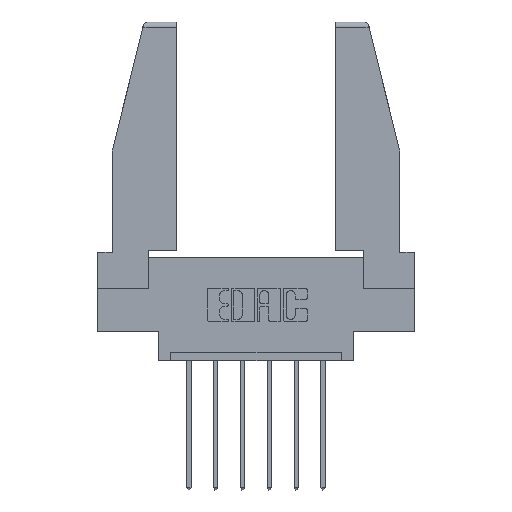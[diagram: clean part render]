
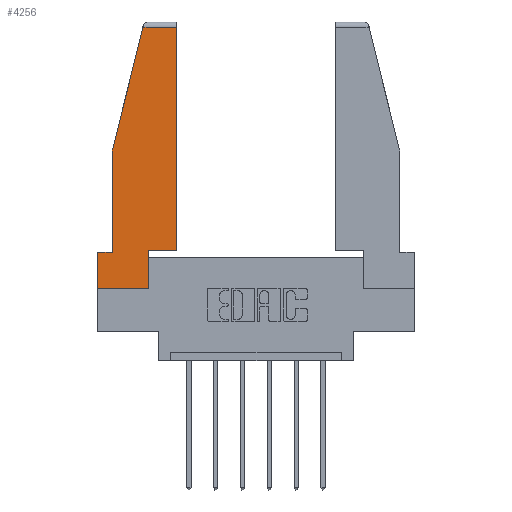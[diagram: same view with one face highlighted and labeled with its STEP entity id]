
A CAD part, top view. The second image highlights one B-rep face of the part: STEP entity #4256.
In plain terms, the highlighted planar face has unit normal (0, 0, 1).
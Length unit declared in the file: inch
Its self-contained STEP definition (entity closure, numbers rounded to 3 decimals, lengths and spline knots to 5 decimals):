
#99 = CARTESIAN_POINT ( 'NONE',  ( 0.297, 0., 0. ) ) ;
#117 = LINE ( 'NONE', #1682, #7533 ) ;
#128 = VERTEX_POINT ( 'NONE', #6214 ) ;
#336 = CARTESIAN_POINT ( 'NONE',  ( 0., 0.21, 0. ) ) ;
#472 = AXIS2_PLACEMENT_3D ( 'NONE', #9961, #860, #3648 ) ;
#632 = CARTESIAN_POINT ( 'NONE',  ( 0.2636, 1.52, 0. ) ) ;
#685 = VECTOR ( 'NONE', #4861, 39.37008 ) ;
#771 = VECTOR ( 'NONE', #7228, 39.37008 ) ;
#847 = CARTESIAN_POINT ( 'NONE',  ( 0.461, 1.52, 0. ) ) ;
#860 = DIRECTION ( 'NONE',  ( 0., 0., 1. ) ) ;
#1025 = VERTEX_POINT ( 'NONE', #632 ) ;
#1047 = EDGE_CURVE ( 'NONE', #10217, #1025, #6096, .T. ) ;
#1245 = DIRECTION ( 'NONE',  ( -1., 0., 0. ) ) ;
#1285 = ORIENTED_EDGE ( 'NONE', *, *, #1887, .T. ) ;
#1404 = ORIENTED_EDGE ( 'NONE', *, *, #4177, .T. ) ;
#1538 = CARTESIAN_POINT ( 'NONE',  ( 0., 1.52, 0. ) ) ;
#1581 = VECTOR ( 'NONE', #1245, 39.37008 ) ;
#1633 = ORIENTED_EDGE ( 'NONE', *, *, #8435, .T. ) ;
#1682 = CARTESIAN_POINT ( 'NONE',  ( 0., 0.21, 0. ) ) ;
#1887 = EDGE_CURVE ( 'NONE', #9279, #9897, #5248, .T. ) ;
#1953 = EDGE_LOOP ( 'NONE', ( #11177, #4930, #1633, #2156, #5743, #11666, #10056, #1285, #1404 ) ) ;
#2156 = ORIENTED_EDGE ( 'NONE', *, *, #6064, .T. ) ;
#2328 = LINE ( 'NONE', #10596, #8303 ) ;
#2685 = DIRECTION ( 'NONE',  ( 0., -1., 0. ) ) ;
#3169 = DIRECTION ( 'NONE',  ( 1., 0., 0. ) ) ;
#3294 = CARTESIAN_POINT ( 'NONE',  ( 0., 0.21, 0. ) ) ;
#3648 = DIRECTION ( 'NONE',  ( 1., 0., 0. ) ) ;
#3787 = DIRECTION ( 'NONE',  ( 0., -1., 0. ) ) ;
#3965 = CARTESIAN_POINT ( 'NONE',  ( 0.297, 0.223, 0. ) ) ;
#3994 = EDGE_CURVE ( 'NONE', #9387, #10217, #2328, .T. ) ;
#4177 = EDGE_CURVE ( 'NONE', #9897, #9387, #7897, .T. ) ;
#4256 = ADVANCED_FACE ( 'NONE', ( #4471 ), #10036, .T. ) ;
#4471 = FACE_OUTER_BOUND ( 'NONE', #1953, .T. ) ;
#4685 = CARTESIAN_POINT ( 'NONE',  ( 0., 0., 0. ) ) ;
#4861 = DIRECTION ( 'NONE',  ( 0., 1., 0. ) ) ;
#4930 = ORIENTED_EDGE ( 'NONE', *, *, #1047, .T. ) ;
#5167 = EDGE_CURVE ( 'NONE', #128, #5883, #8150, .T. ) ;
#5248 = LINE ( 'NONE', #99, #685 ) ;
#5419 = LINE ( 'NONE', #6001, #10674 ) ;
#5514 = CARTESIAN_POINT ( 'NONE',  ( 0.297, 0., 0. ) ) ;
#5559 = DIRECTION ( 'NONE',  ( -1., 0., 0. ) ) ;
#5658 = CARTESIAN_POINT ( 'NONE',  ( 0.461, 0.223, 0. ) ) ;
#5690 = VERTEX_POINT ( 'NONE', #4685 ) ;
#5743 = ORIENTED_EDGE ( 'NONE', *, *, #5167, .T. ) ;
#5883 = VERTEX_POINT ( 'NONE', #3294 ) ;
#6001 = CARTESIAN_POINT ( 'NONE',  ( 0.271, 1.55, 0. ) ) ;
#6064 = EDGE_CURVE ( 'NONE', #8165, #128, #10999, .T. ) ;
#6096 = LINE ( 'NONE', #1538, #6512 ) ;
#6203 = DIRECTION ( 'NONE',  ( 0., 1., 0. ) ) ;
#6214 = CARTESIAN_POINT ( 'NONE',  ( 0.086, 0.21, 0. ) ) ;
#6307 = CARTESIAN_POINT ( 'NONE',  ( 0., 0., 0. ) ) ;
#6512 = VECTOR ( 'NONE', #5559, 39.37008 ) ;
#6668 = EDGE_CURVE ( 'NONE', #5690, #9279, #11415, .T. ) ;
#7228 = DIRECTION ( 'NONE',  ( 1., 0., 0. ) ) ;
#7533 = VECTOR ( 'NONE', #2685, 39.37008 ) ;
#7897 = LINE ( 'NONE', #9686, #10703 ) ;
#8150 = LINE ( 'NONE', #336, #1581 ) ;
#8165 = VERTEX_POINT ( 'NONE', #9210 ) ;
#8303 = VECTOR ( 'NONE', #6203, 39.37008 ) ;
#8435 = EDGE_CURVE ( 'NONE', #1025, #8165, #5419, .T. ) ;
#9210 = CARTESIAN_POINT ( 'NONE',  ( 0.086, 0.8, 0. ) ) ;
#9279 = VERTEX_POINT ( 'NONE', #5514 ) ;
#9363 = EDGE_CURVE ( 'NONE', #5883, #5690, #117, .T. ) ;
#9387 = VERTEX_POINT ( 'NONE', #5658 ) ;
#9686 = CARTESIAN_POINT ( 'NONE',  ( 0.297, 0.223, 0. ) ) ;
#9871 = CARTESIAN_POINT ( 'NONE',  ( 0.086, 0.8, 0. ) ) ;
#9897 = VERTEX_POINT ( 'NONE', #3965 ) ;
#9961 = CARTESIAN_POINT ( 'NONE',  ( 0., 0., 0. ) ) ;
#10036 = PLANE ( 'NONE',  #472 ) ;
#10056 = ORIENTED_EDGE ( 'NONE', *, *, #6668, .T. ) ;
#10217 = VERTEX_POINT ( 'NONE', #847 ) ;
#10378 = DIRECTION ( 'NONE',  ( -0.239, -0.971, 0. ) ) ;
#10596 = CARTESIAN_POINT ( 'NONE',  ( 0.461, 0.223, 0. ) ) ;
#10674 = VECTOR ( 'NONE', #10378, 39.37008 ) ;
#10703 = VECTOR ( 'NONE', #3169, 39.37008 ) ;
#10999 = LINE ( 'NONE', #9871, #11428 ) ;
#11177 = ORIENTED_EDGE ( 'NONE', *, *, #3994, .T. ) ;
#11415 = LINE ( 'NONE', #6307, #771 ) ;
#11428 = VECTOR ( 'NONE', #3787, 39.37008 ) ;
#11666 = ORIENTED_EDGE ( 'NONE', *, *, #9363, .T. ) ;
